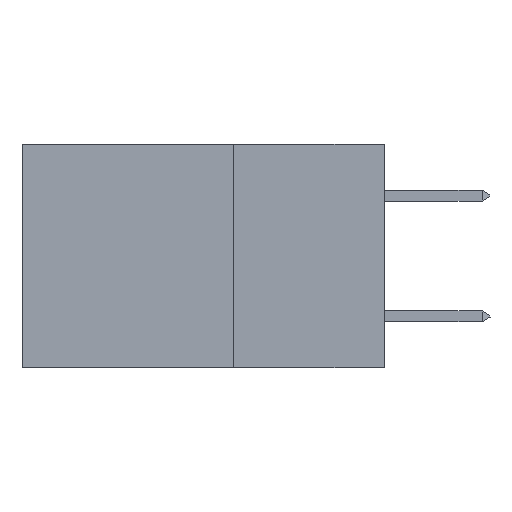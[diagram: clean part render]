
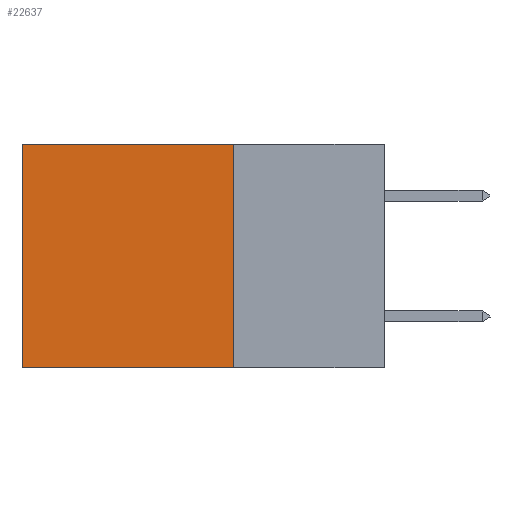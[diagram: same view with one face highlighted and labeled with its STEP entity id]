
A CAD part, left-side view. The second image highlights one B-rep face of the part: STEP entity #22637.
In plain terms, the highlighted planar face has unit normal (-1, 0, 0).
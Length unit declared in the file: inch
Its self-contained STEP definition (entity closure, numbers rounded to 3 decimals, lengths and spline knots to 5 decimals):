
#256 = DIRECTION ( 'NONE',  ( 0., 0., -1. ) ) ;
#978 = CARTESIAN_POINT ( 'NONE',  ( 0.2875, 0.25, 0. ) ) ;
#1569 = ORIENTED_EDGE ( 'NONE', *, *, #10859, .T. ) ;
#1789 = PLANE ( 'NONE',  #4394 ) ;
#2561 = DIRECTION ( 'NONE',  ( 0., 1., 0. ) ) ;
#3000 = CARTESIAN_POINT ( 'NONE',  ( 0.2875, 0.6, 0. ) ) ;
#3210 = LINE ( 'NONE', #13382, #24402 ) ;
#3411 = LINE ( 'NONE', #20051, #25986 ) ;
#3741 = CARTESIAN_POINT ( 'NONE',  ( 0.2875, 0.25, 0. ) ) ;
#4394 = AXIS2_PLACEMENT_3D ( 'NONE', #15196, #17567, #15291 ) ;
#4785 = FACE_OUTER_BOUND ( 'NONE', #6666, .T. ) ;
#5467 = DIRECTION ( 'NONE',  ( 0., 1., 0. ) ) ;
#6178 = LINE ( 'NONE', #3741, #15790 ) ;
#6666 = EDGE_LOOP ( 'NONE', ( #17650, #8083, #26755, #1569 ) ) ;
#8083 = ORIENTED_EDGE ( 'NONE', *, *, #21024, .F. ) ;
#8154 = VERTEX_POINT ( 'NONE', #22150 ) ;
#8700 = EDGE_CURVE ( 'NONE', #20967, #8154, #6178, .T. ) ;
#9230 = LINE ( 'NONE', #28360, #15094 ) ;
#10859 = EDGE_CURVE ( 'NONE', #20967, #21430, #3411, .T. ) ;
#13382 = CARTESIAN_POINT ( 'NONE',  ( 0.2875, 0.25, -0.37 ) ) ;
#15094 = VECTOR ( 'NONE', #256, 39.37008 ) ;
#15196 = CARTESIAN_POINT ( 'NONE',  ( 0.2875, 0.25, 0. ) ) ;
#15291 = DIRECTION ( 'NONE',  ( 0., 0., -1. ) ) ;
#15790 = VECTOR ( 'NONE', #25754, 39.37008 ) ;
#17237 = VERTEX_POINT ( 'NONE', #25133 ) ;
#17567 = DIRECTION ( 'NONE',  ( 1., 0., 0. ) ) ;
#17650 = ORIENTED_EDGE ( 'NONE', *, *, #17789, .T. ) ;
#17789 = EDGE_CURVE ( 'NONE', #21430, #17237, #9230, .T. ) ;
#20051 = CARTESIAN_POINT ( 'NONE',  ( 0.2875, 0.25, 0. ) ) ;
#20967 = VERTEX_POINT ( 'NONE', #978 ) ;
#21024 = EDGE_CURVE ( 'NONE', #8154, #17237, #3210, .T. ) ;
#21430 = VERTEX_POINT ( 'NONE', #3000 ) ;
#22150 = CARTESIAN_POINT ( 'NONE',  ( 0.2875, 0.25, -0.37 ) ) ;
#22637 = ADVANCED_FACE ( 'NONE', ( #4785 ), #1789, .F. ) ;
#24402 = VECTOR ( 'NONE', #2561, 39.37008 ) ;
#25133 = CARTESIAN_POINT ( 'NONE',  ( 0.2875, 0.6, -0.37 ) ) ;
#25754 = DIRECTION ( 'NONE',  ( 0., 0., -1. ) ) ;
#25986 = VECTOR ( 'NONE', #5467, 39.37008 ) ;
#26755 = ORIENTED_EDGE ( 'NONE', *, *, #8700, .F. ) ;
#28360 = CARTESIAN_POINT ( 'NONE',  ( 0.2875, 0.6, 0. ) ) ;
